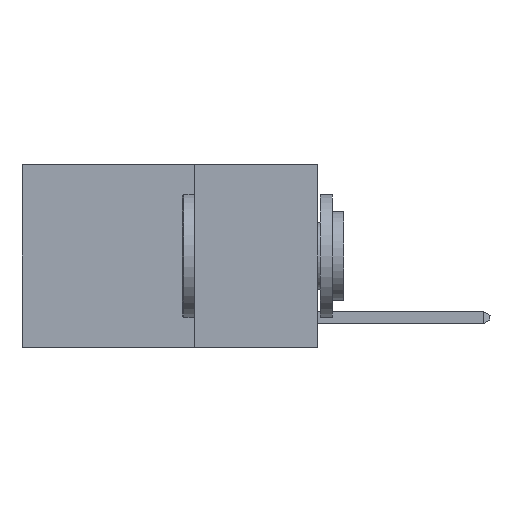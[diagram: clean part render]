
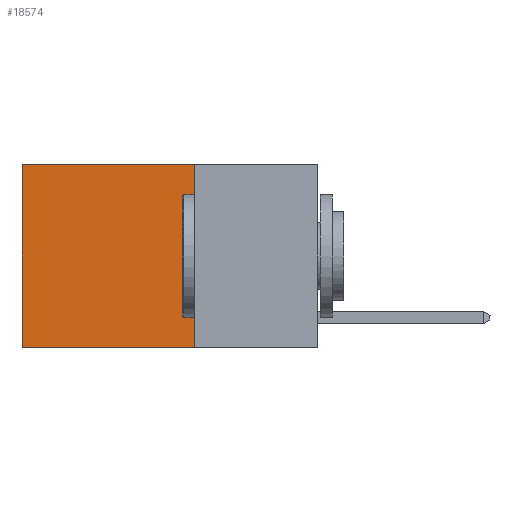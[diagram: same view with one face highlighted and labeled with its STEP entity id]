
A CAD part, left-side view. The second image highlights one B-rep face of the part: STEP entity #18574.
In plain terms, the highlighted planar face has unit normal (-1, 0, 0).
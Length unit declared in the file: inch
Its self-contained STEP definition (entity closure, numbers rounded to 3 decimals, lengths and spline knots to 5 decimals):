
#84 = VERTEX_POINT ( 'NONE', #527 ) ;
#527 = CARTESIAN_POINT ( 'NONE',  ( 0.2625, 0.6, 0. ) ) ;
#1313 = PLANE ( 'NONE',  #1909 ) ;
#1747 = ORIENTED_EDGE ( 'NONE', *, *, #8074, .F. ) ;
#1909 = AXIS2_PLACEMENT_3D ( 'NONE', #5579, #9542, #3768 ) ;
#2198 = LINE ( 'NONE', #10031, #3118 ) ;
#2542 = VECTOR ( 'NONE', #12073, 39.37008 ) ;
#2703 = VECTOR ( 'NONE', #22651, 39.37008 ) ;
#2909 = LINE ( 'NONE', #15192, #13375 ) ;
#3118 = VECTOR ( 'NONE', #19347, 39.37008 ) ;
#3434 = DIRECTION ( 'NONE',  ( 0., 0., -1. ) ) ;
#3768 = DIRECTION ( 'NONE',  ( 0., 0., -1. ) ) ;
#4156 = CARTESIAN_POINT ( 'NONE',  ( 0.2625, 0.25, -0.37 ) ) ;
#5579 = CARTESIAN_POINT ( 'NONE',  ( 0.2625, 0.25, 0. ) ) ;
#7120 = ORIENTED_EDGE ( 'NONE', *, *, #18808, .F. ) ;
#8074 = EDGE_CURVE ( 'NONE', #18546, #23175, #11476, .T. ) ;
#9542 = DIRECTION ( 'NONE',  ( 1., 0., 0. ) ) ;
#10031 = CARTESIAN_POINT ( 'NONE',  ( 0.2625, 0.25, 0. ) ) ;
#11476 = LINE ( 'NONE', #4156, #2542 ) ;
#12073 = DIRECTION ( 'NONE',  ( 0., 1., 0. ) ) ;
#12304 = VERTEX_POINT ( 'NONE', #22420 ) ;
#13375 = VECTOR ( 'NONE', #3434, 39.37008 ) ;
#15108 = ORIENTED_EDGE ( 'NONE', *, *, #18567, .T. ) ;
#15192 = CARTESIAN_POINT ( 'NONE',  ( 0.2625, 0.6, 0. ) ) ;
#15561 = EDGE_CURVE ( 'NONE', #84, #23175, #2909, .T. ) ;
#18546 = VERTEX_POINT ( 'NONE', #19225 ) ;
#18567 = EDGE_CURVE ( 'NONE', #12304, #84, #23032, .T. ) ;
#18574 = ADVANCED_FACE ( 'NONE', ( #24668 ), #1313, .F. ) ;
#18716 = CARTESIAN_POINT ( 'NONE',  ( 0.2625, 0.25, 0. ) ) ;
#18808 = EDGE_CURVE ( 'NONE', #12304, #18546, #2198, .T. ) ;
#19225 = CARTESIAN_POINT ( 'NONE',  ( 0.2625, 0.25, -0.37 ) ) ;
#19347 = DIRECTION ( 'NONE',  ( 0., 0., -1. ) ) ;
#22392 = EDGE_LOOP ( 'NONE', ( #23580, #1747, #7120, #15108 ) ) ;
#22420 = CARTESIAN_POINT ( 'NONE',  ( 0.2625, 0.25, 0. ) ) ;
#22651 = DIRECTION ( 'NONE',  ( 0., 1., 0. ) ) ;
#22675 = CARTESIAN_POINT ( 'NONE',  ( 0.2625, 0.6, -0.37 ) ) ;
#23032 = LINE ( 'NONE', #18716, #2703 ) ;
#23175 = VERTEX_POINT ( 'NONE', #22675 ) ;
#23580 = ORIENTED_EDGE ( 'NONE', *, *, #15561, .T. ) ;
#24668 = FACE_OUTER_BOUND ( 'NONE', #22392, .T. ) ;
